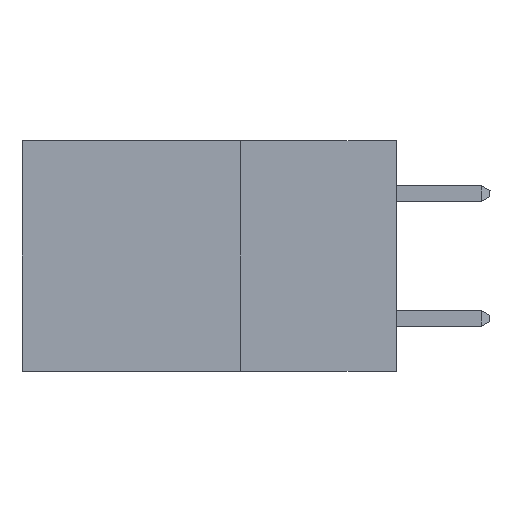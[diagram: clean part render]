
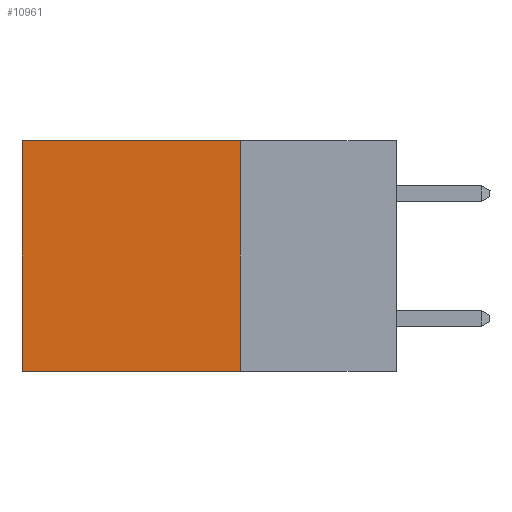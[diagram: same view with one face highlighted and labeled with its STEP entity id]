
A CAD part, left-side view. The second image highlights one B-rep face of the part: STEP entity #10961.
In plain terms, the highlighted planar face has unit normal (-1, 0, 0).
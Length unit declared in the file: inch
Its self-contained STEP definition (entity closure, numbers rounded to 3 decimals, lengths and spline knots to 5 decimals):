
#312 = CARTESIAN_POINT ( 'NONE',  ( 0.298, 0.25, -0.37 ) ) ;
#390 = VECTOR ( 'NONE', #15589, 39.37008 ) ;
#912 = DIRECTION ( 'NONE',  ( 0., 0., -1. ) ) ;
#913 = LINE ( 'NONE', #13985, #390 ) ;
#1400 = LINE ( 'NONE', #11527, #17554 ) ;
#2265 = EDGE_CURVE ( 'NONE', #15233, #16200, #1400, .T. ) ;
#2994 = FACE_OUTER_BOUND ( 'NONE', #4063, .T. ) ;
#3000 = ORIENTED_EDGE ( 'NONE', *, *, #2265, .F. ) ;
#3642 = AXIS2_PLACEMENT_3D ( 'NONE', #5811, #10955, #912 ) ;
#4063 = EDGE_LOOP ( 'NONE', ( #20480, #11233, #3000, #19244 ) ) ;
#5811 = CARTESIAN_POINT ( 'NONE',  ( 0.298, 0.25, 0. ) ) ;
#6152 = DIRECTION ( 'NONE',  ( 0., 1., 0. ) ) ;
#6459 = VECTOR ( 'NONE', #6152, 39.37008 ) ;
#7708 = VECTOR ( 'NONE', #13748, 39.37008 ) ;
#9021 = VERTEX_POINT ( 'NONE', #13231 ) ;
#9186 = PLANE ( 'NONE',  #3642 ) ;
#9722 = VERTEX_POINT ( 'NONE', #14926 ) ;
#10167 = EDGE_CURVE ( 'NONE', #15233, #9021, #16124, .T. ) ;
#10395 = CARTESIAN_POINT ( 'NONE',  ( 0.298, 0.25, 0. ) ) ;
#10955 = DIRECTION ( 'NONE',  ( 1., 0., 0. ) ) ;
#10961 = ADVANCED_FACE ( 'NONE', ( #2994 ), #9186, .F. ) ;
#10987 = LINE ( 'NONE', #11146, #6459 ) ;
#11146 = CARTESIAN_POINT ( 'NONE',  ( 0.298, 0.25, -0.37 ) ) ;
#11233 = ORIENTED_EDGE ( 'NONE', *, *, #21375, .F. ) ;
#11518 = EDGE_CURVE ( 'NONE', #9021, #9722, #913, .T. ) ;
#11527 = CARTESIAN_POINT ( 'NONE',  ( 0.298, 0.25, 0. ) ) ;
#13231 = CARTESIAN_POINT ( 'NONE',  ( 0.298, 0.6, 0. ) ) ;
#13748 = DIRECTION ( 'NONE',  ( 0., 1., 0. ) ) ;
#13985 = CARTESIAN_POINT ( 'NONE',  ( 0.298, 0.6, 0. ) ) ;
#14926 = CARTESIAN_POINT ( 'NONE',  ( 0.298, 0.6, -0.37 ) ) ;
#15233 = VERTEX_POINT ( 'NONE', #17943 ) ;
#15589 = DIRECTION ( 'NONE',  ( 0., 0., -1. ) ) ;
#16124 = LINE ( 'NONE', #10395, #7708 ) ;
#16200 = VERTEX_POINT ( 'NONE', #312 ) ;
#17554 = VECTOR ( 'NONE', #20308, 39.37008 ) ;
#17943 = CARTESIAN_POINT ( 'NONE',  ( 0.298, 0.25, 0. ) ) ;
#19244 = ORIENTED_EDGE ( 'NONE', *, *, #10167, .T. ) ;
#20308 = DIRECTION ( 'NONE',  ( 0., 0., -1. ) ) ;
#20480 = ORIENTED_EDGE ( 'NONE', *, *, #11518, .T. ) ;
#21375 = EDGE_CURVE ( 'NONE', #16200, #9722, #10987, .T. ) ;
